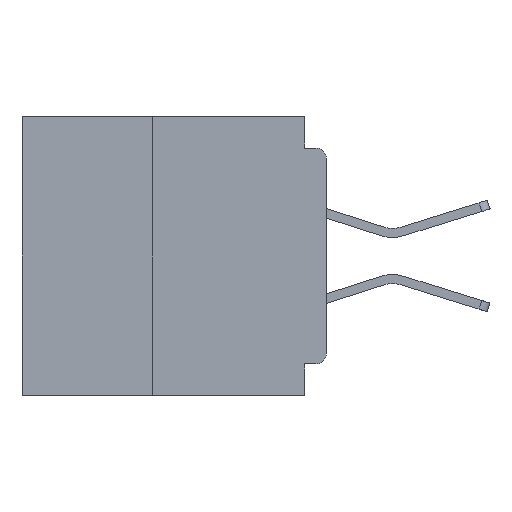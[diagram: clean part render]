
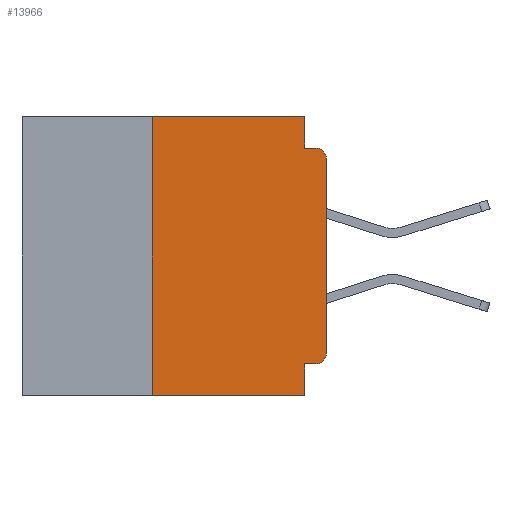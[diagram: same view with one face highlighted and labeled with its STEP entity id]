
A CAD part, left-side view. The second image highlights one B-rep face of the part: STEP entity #13966.
In plain terms, the highlighted planar face has unit normal (-1, 0, 0).
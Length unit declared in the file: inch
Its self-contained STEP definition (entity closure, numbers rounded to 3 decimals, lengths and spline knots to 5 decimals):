
#259 = ORIENTED_EDGE ( 'NONE', *, *, #3899, .T. ) ;
#736 = AXIS2_PLACEMENT_3D ( 'NONE', #44805, #22012, #48610 ) ;
#795 = VECTOR ( 'NONE', #43019, 39.37008 ) ;
#1311 = VECTOR ( 'NONE', #12305, 39.37008 ) ;
#3075 = ORIENTED_EDGE ( 'NONE', *, *, #34661, .T. ) ;
#3111 = CARTESIAN_POINT ( 'NONE',  ( 0., 0.015, -0.355 ) ) ;
#3210 = VECTOR ( 'NONE', #25402, 39.37008 ) ;
#3429 = CARTESIAN_POINT ( 'NONE',  ( 0., 0., -0.355 ) ) ;
#3899 = EDGE_CURVE ( 'NONE', #11015, #24601, #40772, .T. ) ;
#4142 = ORIENTED_EDGE ( 'NONE', *, *, #12029, .F. ) ;
#4641 = CARTESIAN_POINT ( 'NONE',  ( 0., 0.25, -0.4 ) ) ;
#4722 = VERTEX_POINT ( 'NONE', #32657 ) ;
#5292 = VERTEX_POINT ( 'NONE', #28153 ) ;
#5327 = VECTOR ( 'NONE', #30706, 39.37008 ) ;
#5659 = ORIENTED_EDGE ( 'NONE', *, *, #40464, .T. ) ;
#6112 = FACE_OUTER_BOUND ( 'NONE', #30202, .T. ) ;
#6222 = ORIENTED_EDGE ( 'NONE', *, *, #49878, .F. ) ;
#6559 = LINE ( 'NONE', #3429, #5327 ) ;
#8539 = EDGE_CURVE ( 'NONE', #17722, #31835, #6559, .T. ) ;
#8746 = AXIS2_PLACEMENT_3D ( 'NONE', #21169, #47787, #25069 ) ;
#9080 = DIRECTION ( 'NONE',  ( 0., 0., -1. ) ) ;
#9341 = LINE ( 'NONE', #37982, #48921 ) ;
#9727 = CARTESIAN_POINT ( 'NONE',  ( 0., 0.437, 0. ) ) ;
#10247 = CARTESIAN_POINT ( 'NONE',  ( 0., 0.437, 0. ) ) ;
#11015 = VERTEX_POINT ( 'NONE', #11504 ) ;
#11365 = LINE ( 'NONE', #39180, #795 ) ;
#11504 = CARTESIAN_POINT ( 'NONE',  ( 0., 0., -0.34 ) ) ;
#11859 = LINE ( 'NONE', #43013, #1311 ) ;
#12029 = EDGE_CURVE ( 'NONE', #5292, #32156, #13699, .T. ) ;
#12118 = EDGE_CURVE ( 'NONE', #17722, #11015, #41931, .T. ) ;
#12159 = CARTESIAN_POINT ( 'NONE',  ( 0., 0.031, 0. ) ) ;
#12305 = DIRECTION ( 'NONE',  ( 0., 0., -1. ) ) ;
#12804 = EDGE_CURVE ( 'NONE', #4722, #44769, #9341, .T. ) ;
#13699 = LINE ( 'NONE', #9727, #3210 ) ;
#13966 = ADVANCED_FACE ( 'NONE', ( #6112 ), #33401, .F. ) ;
#14190 = DIRECTION ( 'NONE',  ( 1., 0., 0. ) ) ;
#15202 = CARTESIAN_POINT ( 'NONE',  ( 0., 0., 0. ) ) ;
#15628 = LINE ( 'NONE', #43709, #44954 ) ;
#15636 = VERTEX_POINT ( 'NONE', #15719 ) ;
#15719 = CARTESIAN_POINT ( 'NONE',  ( 0., 0.031, -0.4 ) ) ;
#16056 = AXIS2_PLACEMENT_3D ( 'NONE', #10247, #14190, #41027 ) ;
#17003 = VECTOR ( 'NONE', #24147, 39.37008 ) ;
#17722 = VERTEX_POINT ( 'NONE', #3111 ) ;
#18517 = ORIENTED_EDGE ( 'NONE', *, *, #12118, .T. ) ;
#19157 = DIRECTION ( 'NONE',  ( 0., 0., 1. ) ) ;
#21169 = CARTESIAN_POINT ( 'NONE',  ( 0., 0.015, -0.06 ) ) ;
#21844 = EDGE_CURVE ( 'NONE', #31835, #15636, #15628, .T. ) ;
#21923 = ORIENTED_EDGE ( 'NONE', *, *, #8539, .F. ) ;
#22012 = DIRECTION ( 'NONE',  ( -1., 0., 0. ) ) ;
#23746 = VERTEX_POINT ( 'NONE', #25930 ) ;
#24147 = DIRECTION ( 'NONE',  ( 0., 0., 1. ) ) ;
#24236 = CARTESIAN_POINT ( 'NONE',  ( 0., 0.015, -0.045 ) ) ;
#24601 = VERTEX_POINT ( 'NONE', #27366 ) ;
#25069 = DIRECTION ( 'NONE',  ( 0., 0., -1. ) ) ;
#25402 = DIRECTION ( 'NONE',  ( 0., -1., 0. ) ) ;
#25930 = CARTESIAN_POINT ( 'NONE',  ( 0., 0.25, -0.4 ) ) ;
#26693 = DIRECTION ( 'NONE',  ( 0., -1., 0. ) ) ;
#27366 = CARTESIAN_POINT ( 'NONE',  ( 0., 0., -0.06 ) ) ;
#28153 = CARTESIAN_POINT ( 'NONE',  ( 0., 0.25, 0. ) ) ;
#28620 = ORIENTED_EDGE ( 'NONE', *, *, #12804, .F. ) ;
#29500 = VECTOR ( 'NONE', #19157, 39.37008 ) ;
#30202 = EDGE_LOOP ( 'NONE', ( #259, #5659, #28620, #6222, #4142, #47960, #3075, #37079, #21923, #18517 ) ) ;
#30706 = DIRECTION ( 'NONE',  ( 0., 1., 0. ) ) ;
#31835 = VERTEX_POINT ( 'NONE', #40924 ) ;
#32156 = VERTEX_POINT ( 'NONE', #12159 ) ;
#32657 = CARTESIAN_POINT ( 'NONE',  ( 0., 0.031, -0.045 ) ) ;
#33401 = PLANE ( 'NONE',  #16056 ) ;
#34661 = EDGE_CURVE ( 'NONE', #23746, #15636, #11365, .T. ) ;
#37079 = ORIENTED_EDGE ( 'NONE', *, *, #21844, .F. ) ;
#37982 = CARTESIAN_POINT ( 'NONE',  ( 0., 0., -0.045 ) ) ;
#39105 = CIRCLE ( 'NONE', #8746, 0.015 ) ;
#39180 = CARTESIAN_POINT ( 'NONE',  ( 0., 0.437, -0.4 ) ) ;
#39736 = EDGE_CURVE ( 'NONE', #23746, #5292, #47460, .T. ) ;
#40464 = EDGE_CURVE ( 'NONE', #24601, #44769, #39105, .T. ) ;
#40772 = LINE ( 'NONE', #15202, #29500 ) ;
#40924 = CARTESIAN_POINT ( 'NONE',  ( 0., 0.031, -0.355 ) ) ;
#41027 = DIRECTION ( 'NONE',  ( 0., 0., -1. ) ) ;
#41931 = CIRCLE ( 'NONE', #736, 0.015 ) ;
#43013 = CARTESIAN_POINT ( 'NONE',  ( 0., 0.031, 0. ) ) ;
#43019 = DIRECTION ( 'NONE',  ( 0., -1., 0. ) ) ;
#43709 = CARTESIAN_POINT ( 'NONE',  ( 0., 0.031, -0.4 ) ) ;
#44769 = VERTEX_POINT ( 'NONE', #24236 ) ;
#44805 = CARTESIAN_POINT ( 'NONE',  ( 0., 0.015, -0.34 ) ) ;
#44954 = VECTOR ( 'NONE', #9080, 39.37008 ) ;
#47460 = LINE ( 'NONE', #4641, #17003 ) ;
#47787 = DIRECTION ( 'NONE',  ( -1., 0., 0. ) ) ;
#47960 = ORIENTED_EDGE ( 'NONE', *, *, #39736, .F. ) ;
#48610 = DIRECTION ( 'NONE',  ( 0., 0., -1. ) ) ;
#48921 = VECTOR ( 'NONE', #26693, 39.37008 ) ;
#49878 = EDGE_CURVE ( 'NONE', #32156, #4722, #11859, .T. ) ;
